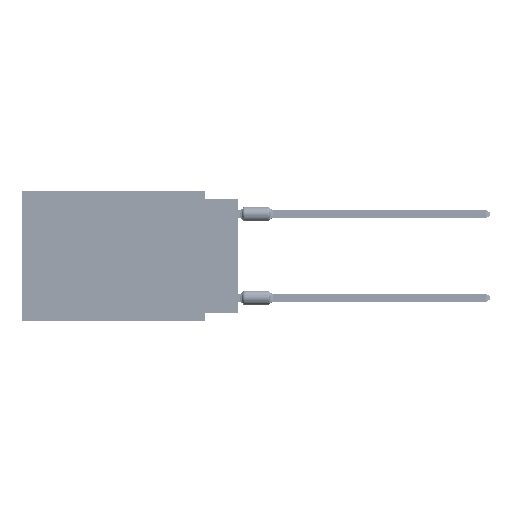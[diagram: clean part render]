
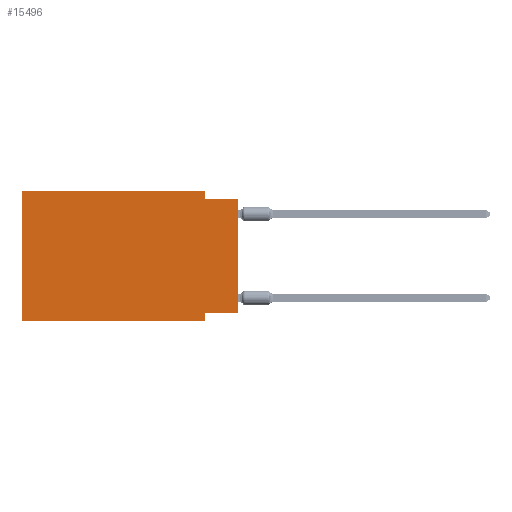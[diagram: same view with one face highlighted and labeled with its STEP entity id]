
A CAD part, left-side view. The second image highlights one B-rep face of the part: STEP entity #15496.
In plain terms, the highlighted planar face has unit normal (-1, 0, 0).
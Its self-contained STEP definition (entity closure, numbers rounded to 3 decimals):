
#375 = EDGE_CURVE ( 'NONE', #25551, #25974, #59165, .T. ) ;
#561 = VERTEX_POINT ( 'NONE', #25928 ) ;
#1358 = FACE_OUTER_BOUND ( 'NONE', #53619, .T. ) ;
#1543 = VECTOR ( 'NONE', #45116, 1000. ) ;
#1835 = EDGE_CURVE ( 'NONE', #47155, #48219, #53617, .T. ) ;
#2006 = VECTOR ( 'NONE', #53938, 1000. ) ;
#2660 = CARTESIAN_POINT ( 'NONE',  ( 0., 0., -9.271 ) ) ;
#2897 = VECTOR ( 'NONE', #5773, 1000. ) ;
#4550 = VECTOR ( 'NONE', #36572, 1000. ) ;
#5773 = DIRECTION ( 'NONE',  ( 0., -1., 0. ) ) ;
#7109 = ORIENTED_EDGE ( 'NONE', *, *, #51861, .F. ) ;
#7131 = DIRECTION ( 'NONE',  ( 0., 0., -1. ) ) ;
#7405 = VECTOR ( 'NONE', #36962, 1000. ) ;
#8187 = LINE ( 'NONE', #29045, #44388 ) ;
#8515 = EDGE_CURVE ( 'NONE', #25974, #561, #45262, .T. ) ;
#9156 = EDGE_CURVE ( 'NONE', #65504, #39483, #42084, .T. ) ;
#10112 = LINE ( 'NONE', #24469, #63402 ) ;
#10916 = CARTESIAN_POINT ( 'NONE',  ( 0., 16.383, 0. ) ) ;
#10986 = EDGE_CURVE ( 'NONE', #53481, #65504, #16684, .T. ) ;
#11831 = CARTESIAN_POINT ( 'NONE',  ( 0., 0., -0.635 ) ) ;
#15496 = ADVANCED_FACE ( 'NONE', ( #1358 ), #38266, .F. ) ;
#16684 = LINE ( 'NONE', #37549, #2006 ) ;
#19618 = CARTESIAN_POINT ( 'NONE',  ( 0., 16.383, -9.906 ) ) ;
#20794 = ORIENTED_EDGE ( 'NONE', *, *, #1835, .F. ) ;
#24065 = EDGE_CURVE ( 'NONE', #25551, #48219, #35219, .T. ) ;
#24469 = CARTESIAN_POINT ( 'NONE',  ( 0., 2.54, 0. ) ) ;
#25551 = VERTEX_POINT ( 'NONE', #2660 ) ;
#25928 = CARTESIAN_POINT ( 'NONE',  ( 0., 2.54, -9.906 ) ) ;
#25974 = VERTEX_POINT ( 'NONE', #65864 ) ;
#27219 = CARTESIAN_POINT ( 'NONE',  ( 0., 2.54, -0.635 ) ) ;
#28689 = ORIENTED_EDGE ( 'NONE', *, *, #9156, .F. ) ;
#29045 = CARTESIAN_POINT ( 'NONE',  ( 0., 16.383, -9.906 ) ) ;
#29807 = ORIENTED_EDGE ( 'NONE', *, *, #24065, .T. ) ;
#30842 = EDGE_CURVE ( 'NONE', #53481, #561, #8187, .T. ) ;
#31486 = CARTESIAN_POINT ( 'NONE',  ( 0., 16.383, 0. ) ) ;
#33462 = CARTESIAN_POINT ( 'NONE',  ( 0., 16.383, 0. ) ) ;
#34180 = CARTESIAN_POINT ( 'NONE',  ( 0., 0., -9.271 ) ) ;
#35219 = LINE ( 'NONE', #56757, #4550 ) ;
#36111 = DIRECTION ( 'NONE',  ( 0., 0., -1. ) ) ;
#36572 = DIRECTION ( 'NONE',  ( 0., 0., 1. ) ) ;
#36962 = DIRECTION ( 'NONE',  ( 0., -1., 0. ) ) ;
#37549 = CARTESIAN_POINT ( 'NONE',  ( 0., 16.383, 0. ) ) ;
#37884 = CARTESIAN_POINT ( 'NONE',  ( 0., 0., -0.635 ) ) ;
#38266 = PLANE ( 'NONE',  #47183 ) ;
#38756 = ORIENTED_EDGE ( 'NONE', *, *, #8515, .F. ) ;
#39483 = VERTEX_POINT ( 'NONE', #66224 ) ;
#42084 = LINE ( 'NONE', #31486, #7405 ) ;
#42712 = ORIENTED_EDGE ( 'NONE', *, *, #10986, .F. ) ;
#42900 = VECTOR ( 'NONE', #45599, 1000. ) ;
#44388 = VECTOR ( 'NONE', #45456, 1000. ) ;
#45116 = DIRECTION ( 'NONE',  ( 0., 1., 0. ) ) ;
#45262 = LINE ( 'NONE', #45942, #42900 ) ;
#45456 = DIRECTION ( 'NONE',  ( 0., -1., 0. ) ) ;
#45599 = DIRECTION ( 'NONE',  ( 0., 0., -1. ) ) ;
#45942 = CARTESIAN_POINT ( 'NONE',  ( 0., 2.54, -9.906 ) ) ;
#47155 = VERTEX_POINT ( 'NONE', #27219 ) ;
#47183 = AXIS2_PLACEMENT_3D ( 'NONE', #33462, #48522, #7131 ) ;
#48219 = VERTEX_POINT ( 'NONE', #11831 ) ;
#48522 = DIRECTION ( 'NONE',  ( 1., 0., 0. ) ) ;
#51861 = EDGE_CURVE ( 'NONE', #39483, #47155, #10112, .T. ) ;
#53481 = VERTEX_POINT ( 'NONE', #19618 ) ;
#53617 = LINE ( 'NONE', #37884, #2897 ) ;
#53619 = EDGE_LOOP ( 'NONE', ( #29807, #20794, #7109, #28689, #42712, #55666, #38756, #58192 ) ) ;
#53938 = DIRECTION ( 'NONE',  ( 0., 0., 1. ) ) ;
#55666 = ORIENTED_EDGE ( 'NONE', *, *, #30842, .T. ) ;
#56757 = CARTESIAN_POINT ( 'NONE',  ( 0., 0., 0. ) ) ;
#58192 = ORIENTED_EDGE ( 'NONE', *, *, #375, .F. ) ;
#59165 = LINE ( 'NONE', #34180, #1543 ) ;
#63402 = VECTOR ( 'NONE', #36111, 1000. ) ;
#65504 = VERTEX_POINT ( 'NONE', #10916 ) ;
#65864 = CARTESIAN_POINT ( 'NONE',  ( 0., 2.54, -9.271 ) ) ;
#66224 = CARTESIAN_POINT ( 'NONE',  ( 0., 2.54, 0. ) ) ;
